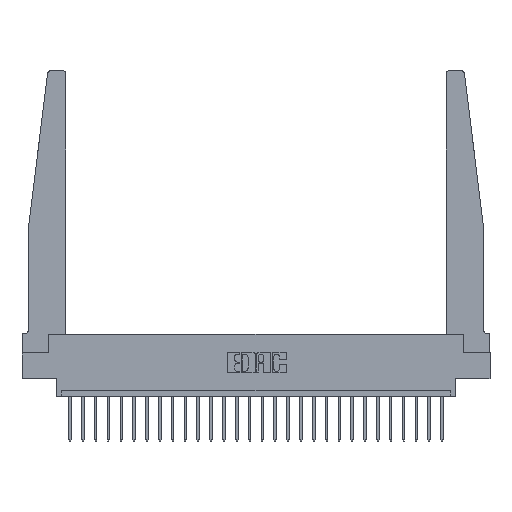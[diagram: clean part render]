
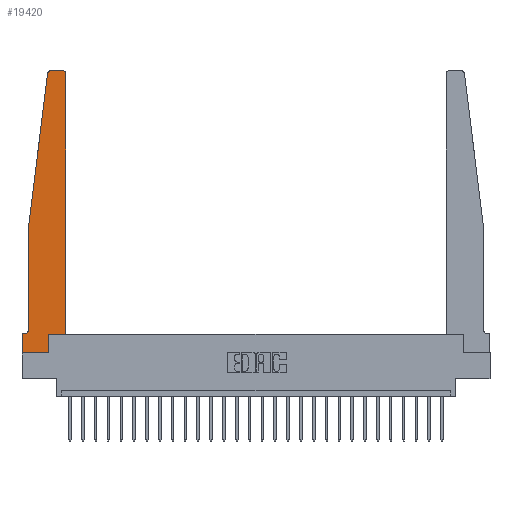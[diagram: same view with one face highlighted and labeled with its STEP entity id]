
A CAD part, top view. The second image highlights one B-rep face of the part: STEP entity #19420.
In plain terms, the highlighted planar face has unit normal (0, 0, 1).
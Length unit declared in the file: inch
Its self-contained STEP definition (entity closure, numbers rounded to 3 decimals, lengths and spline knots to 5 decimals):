
#160 = FACE_OUTER_BOUND ( 'NONE', #19961, .T. ) ;
#409 = VECTOR ( 'NONE', #2363, 39.37008 ) ;
#732 = LINE ( 'NONE', #9735, #24085 ) ;
#1411 = ORIENTED_EDGE ( 'NONE', *, *, #17098, .T. ) ;
#2165 = CARTESIAN_POINT ( 'NONE',  ( 0.27653, 2.75, 0.37 ) ) ;
#2227 = CIRCLE ( 'NONE', #5511, 0.03 ) ;
#2363 = DIRECTION ( 'NONE',  ( 1., 0., 0. ) ) ;
#2699 = AXIS2_PLACEMENT_3D ( 'NONE', #6277, #11988, #13901 ) ;
#2761 = EDGE_CURVE ( 'NONE', #17946, #21350, #3931, .T. ) ;
#3173 = VERTEX_POINT ( 'NONE', #18372 ) ;
#3626 = CIRCLE ( 'NONE', #20567, 0.05 ) ;
#3797 = DIRECTION ( 'NONE',  ( -1., 0., 0. ) ) ;
#3807 = VECTOR ( 'NONE', #20152, 39.37008 ) ;
#3931 = LINE ( 'NONE', #20951, #18192 ) ;
#4031 = DIRECTION ( 'NONE',  ( 0., 1., 0. ) ) ;
#4422 = DIRECTION ( 'NONE',  ( 0., 0., 1. ) ) ;
#4497 = DIRECTION ( 'NONE',  ( 1., 0., 0. ) ) ;
#4507 = DIRECTION ( 'NONE',  ( 1., 0., 0. ) ) ;
#4596 = AXIS2_PLACEMENT_3D ( 'NONE', #24680, #13054, #11471 ) ;
#4854 = VERTEX_POINT ( 'NONE', #19142 ) ;
#5178 = VECTOR ( 'NONE', #22375, 39.37008 ) ;
#5511 = AXIS2_PLACEMENT_3D ( 'NONE', #16016, #4422, #4507 ) ;
#5712 = EDGE_CURVE ( 'NONE', #10533, #11834, #11761, .T. ) ;
#5942 = VERTEX_POINT ( 'NONE', #10398 ) ;
#5960 = DIRECTION ( 'NONE',  ( 0., 1., 0. ) ) ;
#6277 = CARTESIAN_POINT ( 'NONE',  ( 0.27653, 2.72, 0.37 ) ) ;
#6352 = ORIENTED_EDGE ( 'NONE', *, *, #13695, .T. ) ;
#6568 = EDGE_CURVE ( 'NONE', #19114, #24579, #7739, .T. ) ;
#6877 = CARTESIAN_POINT ( 'NONE',  ( 0., 0., 0.37 ) ) ;
#7190 = PLANE ( 'NONE',  #4596 ) ;
#7739 = LINE ( 'NONE', #14927, #14379 ) ;
#7775 = CARTESIAN_POINT ( 'NONE',  ( 0.065, 0.1875, 0.37 ) ) ;
#7817 = CARTESIAN_POINT ( 'NONE',  ( 0.2605, 0.18, 0.37 ) ) ;
#8075 = ORIENTED_EDGE ( 'NONE', *, *, #21456, .T. ) ;
#8304 = CARTESIAN_POINT ( 'NONE',  ( 0.425, 0.18, 0.37 ) ) ;
#9735 = CARTESIAN_POINT ( 'NONE',  ( 0.425, 0.18, 0.37 ) ) ;
#10006 = ORIENTED_EDGE ( 'NONE', *, *, #20955, .T. ) ;
#10368 = ORIENTED_EDGE ( 'NONE', *, *, #23378, .T. ) ;
#10398 = CARTESIAN_POINT ( 'NONE',  ( 0., 0.1875, 0.37 ) ) ;
#10439 = ORIENTED_EDGE ( 'NONE', *, *, #14651, .T. ) ;
#10533 = VERTEX_POINT ( 'NONE', #17436 ) ;
#10849 = CARTESIAN_POINT ( 'NONE',  ( 0.065, 1.25, 0.37 ) ) ;
#11424 = DIRECTION ( 'NONE',  ( 0., -1., 0. ) ) ;
#11471 = DIRECTION ( 'NONE',  ( 1., 0., 0. ) ) ;
#11604 = VECTOR ( 'NONE', #5960, 39.37008 ) ;
#11761 = LINE ( 'NONE', #23746, #19889 ) ;
#11834 = VERTEX_POINT ( 'NONE', #22786 ) ;
#11988 = DIRECTION ( 'NONE',  ( 0., 0., 1. ) ) ;
#12097 = ORIENTED_EDGE ( 'NONE', *, *, #5712, .T. ) ;
#12328 = LINE ( 'NONE', #18385, #3807 ) ;
#12964 = CARTESIAN_POINT ( 'NONE',  ( 0.2605, 0.18, 0.37 ) ) ;
#13054 = DIRECTION ( 'NONE',  ( 0., 0., 1. ) ) ;
#13695 = EDGE_CURVE ( 'NONE', #21433, #17946, #12328, .T. ) ;
#13901 = DIRECTION ( 'NONE',  ( 1., 0., 0. ) ) ;
#14156 = CARTESIAN_POINT ( 'NONE',  ( 0.015, 0.2375, 0.37 ) ) ;
#14379 = VECTOR ( 'NONE', #16716, 39.37008 ) ;
#14554 = EDGE_CURVE ( 'NONE', #19613, #3173, #732, .T. ) ;
#14651 = EDGE_CURVE ( 'NONE', #3173, #19114, #2227, .T. ) ;
#14927 = CARTESIAN_POINT ( 'NONE',  ( 0.25, 2.75, 0.37 ) ) ;
#14948 = ORIENTED_EDGE ( 'NONE', *, *, #2761, .T. ) ;
#16016 = CARTESIAN_POINT ( 'NONE',  ( 0.395, 2.72, 0.37 ) ) ;
#16097 = ORIENTED_EDGE ( 'NONE', *, *, #16121, .T. ) ;
#16107 = DIRECTION ( 'NONE',  ( -1., 0., 0. ) ) ;
#16121 = EDGE_CURVE ( 'NONE', #11834, #16268, #16706, .T. ) ;
#16268 = VERTEX_POINT ( 'NONE', #12964 ) ;
#16706 = LINE ( 'NONE', #7817, #11604 ) ;
#16716 = DIRECTION ( 'NONE',  ( -1., 0., 0. ) ) ;
#16903 = ORIENTED_EDGE ( 'NONE', *, *, #14554, .T. ) ;
#17098 = EDGE_CURVE ( 'NONE', #5942, #10533, #21232, .T. ) ;
#17436 = CARTESIAN_POINT ( 'NONE',  ( 0., 0., 0.37 ) ) ;
#17680 = VECTOR ( 'NONE', #3797, 39.37008 ) ;
#17946 = VERTEX_POINT ( 'NONE', #10849 ) ;
#18115 = CARTESIAN_POINT ( 'NONE',  ( 0.425, 0.18, 0.37 ) ) ;
#18192 = VECTOR ( 'NONE', #11424, 39.37008 ) ;
#18372 = CARTESIAN_POINT ( 'NONE',  ( 0.425, 2.72, 0.37 ) ) ;
#18385 = CARTESIAN_POINT ( 'NONE',  ( 0.065, 1.25, 0.37 ) ) ;
#18568 = CIRCLE ( 'NONE', #2699, 0.03 ) ;
#19114 = VERTEX_POINT ( 'NONE', #24092 ) ;
#19142 = CARTESIAN_POINT ( 'NONE',  ( 0.015, 0.1875, 0.37 ) ) ;
#19420 = ADVANCED_FACE ( 'NONE', ( #160 ), #7190, .T. ) ;
#19460 = CARTESIAN_POINT ( 'NONE',  ( 0.24675, 2.72367, 0.37 ) ) ;
#19613 = VERTEX_POINT ( 'NONE', #18115 ) ;
#19889 = VECTOR ( 'NONE', #4497, 39.37008 ) ;
#19961 = EDGE_LOOP ( 'NONE', ( #21964, #10006, #6352, #14948, #10368, #8075, #1411, #12097, #16097, #24681, #16903, #10439 ) ) ;
#20152 = DIRECTION ( 'NONE',  ( -0.122, -0.992, 0. ) ) ;
#20567 = AXIS2_PLACEMENT_3D ( 'NONE', #14156, #24016, #16107 ) ;
#20951 = CARTESIAN_POINT ( 'NONE',  ( 0.065, 1.25, 0.37 ) ) ;
#20955 = EDGE_CURVE ( 'NONE', #24579, #21433, #18568, .T. ) ;
#21232 = LINE ( 'NONE', #6877, #5178 ) ;
#21350 = VERTEX_POINT ( 'NONE', #24772 ) ;
#21433 = VERTEX_POINT ( 'NONE', #19460 ) ;
#21456 = EDGE_CURVE ( 'NONE', #4854, #5942, #22226, .T. ) ;
#21964 = ORIENTED_EDGE ( 'NONE', *, *, #6568, .T. ) ;
#22226 = LINE ( 'NONE', #7775, #17680 ) ;
#22375 = DIRECTION ( 'NONE',  ( 0., -1., 0. ) ) ;
#22786 = CARTESIAN_POINT ( 'NONE',  ( 0.2605, 0., 0.37 ) ) ;
#23378 = EDGE_CURVE ( 'NONE', #21350, #4854, #3626, .T. ) ;
#23746 = CARTESIAN_POINT ( 'NONE',  ( 0., 0., 0.37 ) ) ;
#23976 = EDGE_CURVE ( 'NONE', #16268, #19613, #25019, .T. ) ;
#24016 = DIRECTION ( 'NONE',  ( 0., 0., -1. ) ) ;
#24085 = VECTOR ( 'NONE', #4031, 39.37008 ) ;
#24092 = CARTESIAN_POINT ( 'NONE',  ( 0.395, 2.75, 0.37 ) ) ;
#24579 = VERTEX_POINT ( 'NONE', #2165 ) ;
#24680 = CARTESIAN_POINT ( 'NONE',  ( 0., 0.1875, 0.37 ) ) ;
#24681 = ORIENTED_EDGE ( 'NONE', *, *, #23976, .T. ) ;
#24772 = CARTESIAN_POINT ( 'NONE',  ( 0.065, 0.2375, 0.37 ) ) ;
#25019 = LINE ( 'NONE', #8304, #409 ) ;
